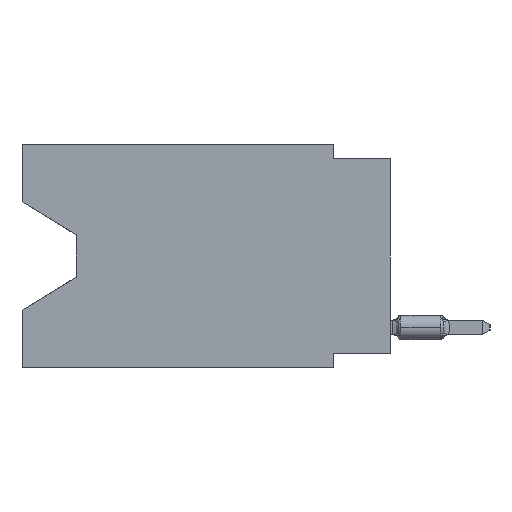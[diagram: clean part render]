
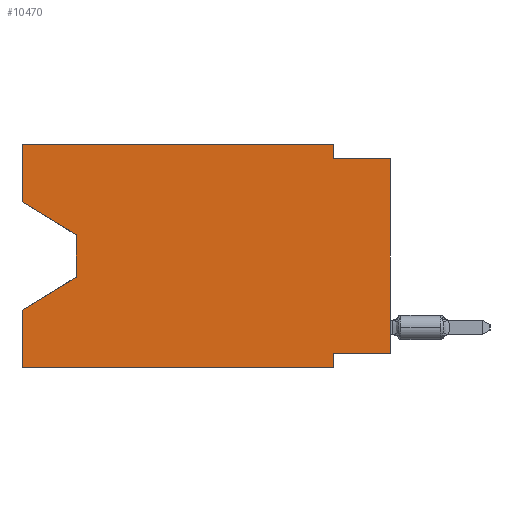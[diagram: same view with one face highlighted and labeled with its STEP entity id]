
A CAD part, left-side view. The second image highlights one B-rep face of the part: STEP entity #10470.
In plain terms, the highlighted planar face has unit normal (-1, 0, 0).
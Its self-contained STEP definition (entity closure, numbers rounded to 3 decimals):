
#785 = VECTOR ( 'NONE', #76472, 1000. ) ;
#2216 = ORIENTED_EDGE ( 'NONE', *, *, #9482, .F. ) ;
#3717 = ORIENTED_EDGE ( 'NONE', *, *, #55613, .F. ) ;
#3829 = VECTOR ( 'NONE', #33555, 1000. ) ;
#4302 = CARTESIAN_POINT ( 'NONE',  ( 0., 2.54, -9.271 ) ) ;
#4663 = LINE ( 'NONE', #70233, #785 ) ;
#5069 = CARTESIAN_POINT ( 'NONE',  ( 0., 13.97, -4.013 ) ) ;
#5731 = CARTESIAN_POINT ( 'NONE',  ( 0., 16.383, -7.36 ) ) ;
#5972 = VECTOR ( 'NONE', #27870, 1000. ) ;
#6191 = CARTESIAN_POINT ( 'NONE',  ( 0., 13.97, -5.893 ) ) ;
#7084 = ORIENTED_EDGE ( 'NONE', *, *, #49911, .T. ) ;
#7300 = VECTOR ( 'NONE', #65441, 1000. ) ;
#9482 = EDGE_CURVE ( 'NONE', #67122, #70898, #65443, .T. ) ;
#9737 = CARTESIAN_POINT ( 'NONE',  ( 0., 13.97, -5.893 ) ) ;
#10152 = ORIENTED_EDGE ( 'NONE', *, *, #24232, .F. ) ;
#10280 = ORIENTED_EDGE ( 'NONE', *, *, #56515, .F. ) ;
#10390 = CARTESIAN_POINT ( 'NONE',  ( 0., 2.54, -9.906 ) ) ;
#10448 = LINE ( 'NONE', #51024, #58964 ) ;
#10470 = ADVANCED_FACE ( 'NONE', ( #67840 ), #31937, .F. ) ;
#10813 = CARTESIAN_POINT ( 'NONE',  ( 0., 16.383, 0. ) ) ;
#11397 = CARTESIAN_POINT ( 'NONE',  ( 0., 0., -9.271 ) ) ;
#13219 = CARTESIAN_POINT ( 'NONE',  ( 0., 16.383, 0. ) ) ;
#14055 = DIRECTION ( 'NONE',  ( 0., 0., -1. ) ) ;
#16437 = ORIENTED_EDGE ( 'NONE', *, *, #28499, .F. ) ;
#18191 = LINE ( 'NONE', #59191, #7300 ) ;
#18713 = VERTEX_POINT ( 'NONE', #30665 ) ;
#19119 = EDGE_CURVE ( 'NONE', #67122, #61691, #65702, .T. ) ;
#21744 = DIRECTION ( 'NONE',  ( 0., 0., -1. ) ) ;
#22137 = DIRECTION ( 'NONE',  ( 0., -0.855, -0.519 ) ) ;
#22434 = ORIENTED_EDGE ( 'NONE', *, *, #19119, .T. ) ;
#23238 = EDGE_CURVE ( 'NONE', #32554, #18713, #33350, .T. ) ;
#24232 = EDGE_CURVE ( 'NONE', #71890, #65221, #18191, .T. ) ;
#24439 = DIRECTION ( 'NONE',  ( 0., 0., 1. ) ) ;
#27870 = DIRECTION ( 'NONE',  ( 0., -1., 0. ) ) ;
#28499 = EDGE_CURVE ( 'NONE', #30446, #64312, #30731, .T. ) ;
#30181 = VECTOR ( 'NONE', #24439, 1000. ) ;
#30446 = VERTEX_POINT ( 'NONE', #11397 ) ;
#30665 = CARTESIAN_POINT ( 'NONE',  ( 0., 0., -0.635 ) ) ;
#30731 = LINE ( 'NONE', #54518, #31614 ) ;
#31614 = VECTOR ( 'NONE', #60772, 1000. ) ;
#31937 = PLANE ( 'NONE',  #35188 ) ;
#32554 = VERTEX_POINT ( 'NONE', #50135 ) ;
#33350 = LINE ( 'NONE', #39970, #5972 ) ;
#33555 = DIRECTION ( 'NONE',  ( 0., 0.855, -0.519 ) ) ;
#34135 = CARTESIAN_POINT ( 'NONE',  ( 0., 13.97, -4.013 ) ) ;
#34214 = LINE ( 'NONE', #47059, #46335 ) ;
#35188 = AXIS2_PLACEMENT_3D ( 'NONE', #13219, #61601, #37008 ) ;
#36184 = CARTESIAN_POINT ( 'NONE',  ( 0., 16.383, -2.546 ) ) ;
#37008 = DIRECTION ( 'NONE',  ( 0., 0., -1. ) ) ;
#38220 = CARTESIAN_POINT ( 'NONE',  ( 0., 2.54, 0. ) ) ;
#39286 = CARTESIAN_POINT ( 'NONE',  ( 0., 16.383, 0. ) ) ;
#39295 = LINE ( 'NONE', #56477, #76825 ) ;
#39970 = CARTESIAN_POINT ( 'NONE',  ( 0., 0., -0.635 ) ) ;
#41497 = ORIENTED_EDGE ( 'NONE', *, *, #64390, .T. ) ;
#42872 = ORIENTED_EDGE ( 'NONE', *, *, #50666, .T. ) ;
#45249 = LINE ( 'NONE', #9737, #3829 ) ;
#45355 = ORIENTED_EDGE ( 'NONE', *, *, #23238, .F. ) ;
#46335 = VECTOR ( 'NONE', #58014, 1000. ) ;
#46433 = LINE ( 'NONE', #5069, #65034 ) ;
#47059 = CARTESIAN_POINT ( 'NONE',  ( 0., 0., 0. ) ) ;
#48393 = LINE ( 'NONE', #38220, #52460 ) ;
#49183 = EDGE_CURVE ( 'NONE', #65221, #32554, #48393, .T. ) ;
#49911 = EDGE_CURVE ( 'NONE', #30446, #18713, #34214, .T. ) ;
#50135 = CARTESIAN_POINT ( 'NONE',  ( 0., 2.54, -0.635 ) ) ;
#50666 = EDGE_CURVE ( 'NONE', #67668, #70898, #45249, .T. ) ;
#51024 = CARTESIAN_POINT ( 'NONE',  ( 0., 16.383, -2.546 ) ) ;
#51588 = VERTEX_POINT ( 'NONE', #34135 ) ;
#52460 = VECTOR ( 'NONE', #14055, 1000. ) ;
#54109 = ORIENTED_EDGE ( 'NONE', *, *, #49183, .F. ) ;
#54518 = CARTESIAN_POINT ( 'NONE',  ( 0., 0., -9.271 ) ) ;
#55613 = EDGE_CURVE ( 'NONE', #76799, #71890, #4663, .T. ) ;
#56477 = CARTESIAN_POINT ( 'NONE',  ( 0., 2.54, -9.906 ) ) ;
#56515 = EDGE_CURVE ( 'NONE', #64312, #61691, #39295, .T. ) ;
#56850 = ORIENTED_EDGE ( 'NONE', *, *, #70730, .T. ) ;
#57190 = VECTOR ( 'NONE', #61000, 1000. ) ;
#58014 = DIRECTION ( 'NONE',  ( 0., 0., 1. ) ) ;
#58964 = VECTOR ( 'NONE', #22137, 1000. ) ;
#59191 = CARTESIAN_POINT ( 'NONE',  ( 0., 16.383, 0. ) ) ;
#59705 = DIRECTION ( 'NONE',  ( 0., 0., -1. ) ) ;
#60772 = DIRECTION ( 'NONE',  ( 0., 1., 0. ) ) ;
#61000 = DIRECTION ( 'NONE',  ( 0., -1., 0. ) ) ;
#61601 = DIRECTION ( 'NONE',  ( 1., 0., 0. ) ) ;
#61691 = VERTEX_POINT ( 'NONE', #10390 ) ;
#62118 = CARTESIAN_POINT ( 'NONE',  ( 0., 16.383, -9.906 ) ) ;
#64312 = VERTEX_POINT ( 'NONE', #4302 ) ;
#64390 = EDGE_CURVE ( 'NONE', #51588, #67668, #46433, .T. ) ;
#65034 = VECTOR ( 'NONE', #59705, 1000. ) ;
#65221 = VERTEX_POINT ( 'NONE', #76688 ) ;
#65441 = DIRECTION ( 'NONE',  ( 0., -1., 0. ) ) ;
#65443 = LINE ( 'NONE', #10813, #30181 ) ;
#65702 = LINE ( 'NONE', #66483, #57190 ) ;
#66483 = CARTESIAN_POINT ( 'NONE',  ( 0., 16.383, -9.906 ) ) ;
#66923 = EDGE_LOOP ( 'NONE', ( #56850, #41497, #42872, #2216, #22434, #10280, #16437, #7084, #45355, #54109, #10152, #3717 ) ) ;
#67122 = VERTEX_POINT ( 'NONE', #62118 ) ;
#67668 = VERTEX_POINT ( 'NONE', #6191 ) ;
#67840 = FACE_OUTER_BOUND ( 'NONE', #66923, .T. ) ;
#70233 = CARTESIAN_POINT ( 'NONE',  ( 0., 16.383, 0. ) ) ;
#70730 = EDGE_CURVE ( 'NONE', #76799, #51588, #10448, .T. ) ;
#70898 = VERTEX_POINT ( 'NONE', #5731 ) ;
#71890 = VERTEX_POINT ( 'NONE', #39286 ) ;
#76472 = DIRECTION ( 'NONE',  ( 0., 0., 1. ) ) ;
#76688 = CARTESIAN_POINT ( 'NONE',  ( 0., 2.54, 0. ) ) ;
#76799 = VERTEX_POINT ( 'NONE', #36184 ) ;
#76825 = VECTOR ( 'NONE', #21744, 1000. ) ;
